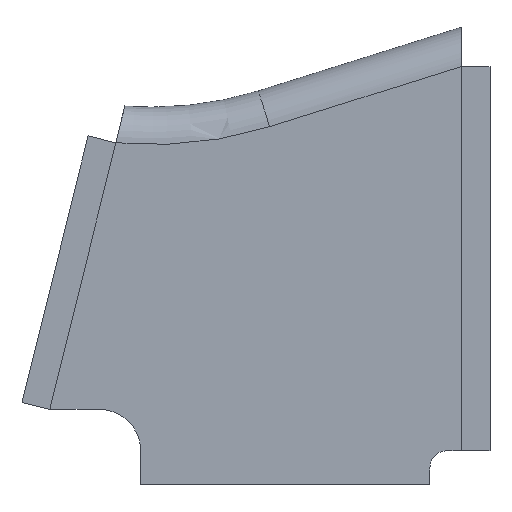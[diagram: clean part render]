
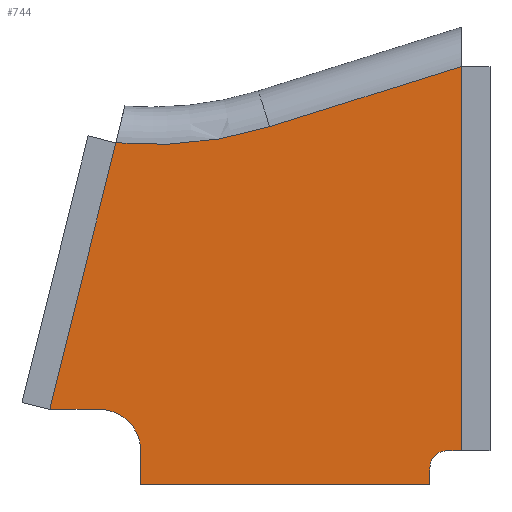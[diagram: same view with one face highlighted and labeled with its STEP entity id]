
A CAD part, front view. The second image highlights one B-rep face of the part: STEP entity #744.
In plain terms, the highlighted planar face has unit normal (0, -1, 0).
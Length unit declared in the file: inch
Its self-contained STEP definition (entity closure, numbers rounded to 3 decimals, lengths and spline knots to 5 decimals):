
#8 = CARTESIAN_POINT ( 'NONE',  ( 0.16386, 0., -3.5792 ) ) ;
#11 = CARTESIAN_POINT ( 'NONE',  ( 3.19927, 0., -3.97455 ) ) ;
#14 = LINE ( 'NONE', #32, #775 ) ;
#19 = DIRECTION ( 'NONE',  ( 0., 0., -1. ) ) ;
#20 = LINE ( 'NONE', #21, #785 ) ;
#21 = CARTESIAN_POINT ( 'NONE',  ( 0., 0., -3.97455 ) ) ;
#23 = CARTESIAN_POINT ( 'NONE',  ( -0.31259, 0., -3.18386 ) ) ;
#27 = LINE ( 'NONE', #37, #770 ) ;
#28 = DIRECTION ( 'NONE',  ( 1., 0., 0. ) ) ;
#32 = CARTESIAN_POINT ( 'NONE',  ( 0.16386, 0., 0. ) ) ;
#33 = CARTESIAN_POINT ( 'NONE',  ( -0.78905, 0., -3.18386 ) ) ;
#37 = CARTESIAN_POINT ( 'NONE',  ( 0., 0., -3.18386 ) ) ;
#40 = DIRECTION ( 'NONE',  ( 0., 1., 0. ) ) ;
#43 = DIRECTION ( 'NONE',  ( 1., 0., 0. ) ) ;
#44 = LINE ( 'NONE', #68, #783 ) ;
#51 = DIRECTION ( 'NONE',  ( 0., 0., 1. ) ) ;
#57 = CARTESIAN_POINT ( 'NONE',  ( -0.27204, 0., -3.61976 ) ) ;
#65 = CARTESIAN_POINT ( 'NONE',  ( 3.37051, 0., -3.791 ) ) ;
#66 = DIRECTION ( 'NONE',  ( 0., 0., 1. ) ) ;
#68 = CARTESIAN_POINT ( 'NONE',  ( 3.19927, 0., 0. ) ) ;
#79 = CARTESIAN_POINT ( 'NONE',  ( 0., 0., 0. ) ) ;
#83 = LINE ( 'NONE', #79, #784 ) ;
#86 = DIRECTION ( 'NONE',  ( -0.241, 0., -0.971 ) ) ;
#93 = DIRECTION ( 'NONE',  ( 0., 0., 1. ) ) ;
#100 = DIRECTION ( 'NONE',  ( 0., -1., 0. ) ) ;
#141 = LINE ( 'NONE', #151, #795 ) ;
#142 = DIRECTION ( 'NONE',  ( -0.954, 0., -0.299 ) ) ;
#148 = DIRECTION ( 'NONE',  ( 0., 1., 0. ) ) ;
#151 = CARTESIAN_POINT ( 'NONE',  ( 0.1982, 0., -0.63165 ) ) ;
#153 = CARTESIAN_POINT ( 'NONE',  ( 0.293, 0., 3.68369 ) ) ;
#159 = DIRECTION ( 'NONE',  ( 0., 0., 1. ) ) ;
#230 = CARTESIAN_POINT ( 'NONE',  ( 0., 0., -3.61976 ) ) ;
#232 = LINE ( 'NONE', #260, #855 ) ;
#244 = LINE ( 'NONE', #230, #815 ) ;
#254 = DIRECTION ( 'NONE',  ( 0., 0., -1. ) ) ;
#257 = DIRECTION ( 'NONE',  ( 1., 0., 0. ) ) ;
#260 = CARTESIAN_POINT ( 'NONE',  ( 3.52943, 0., 0. ) ) ;
#331 = PLANE ( 'NONE',  #862 ) ;
#332 = CARTESIAN_POINT ( 'NONE',  ( 0., 0., 0. ) ) ;
#337 = DIRECTION ( 'NONE',  ( 0., 0., 1. ) ) ;
#340 = DIRECTION ( 'NONE',  ( 0., 1., 0. ) ) ;
#454 = ORIENTED_EDGE ( 'NONE', *, *, #713, .T. ) ;
#459 = ORIENTED_EDGE ( 'NONE', *, *, #717, .F. ) ;
#463 = ORIENTED_EDGE ( 'NONE', *, *, #676, .F. ) ;
#469 = ORIENTED_EDGE ( 'NONE', *, *, #674, .T. ) ;
#472 = ORIENTED_EDGE ( 'NONE', *, *, #667, .T. ) ;
#474 = ORIENTED_EDGE ( 'NONE', *, *, #657, .T. ) ;
#475 = ORIENTED_EDGE ( 'NONE', *, *, #659, .T. ) ;
#477 = ORIENTED_EDGE ( 'NONE', *, *, #661, .T. ) ;
#494 = ORIENTED_EDGE ( 'NONE', *, *, #689, .T. ) ;
#496 = ORIENTED_EDGE ( 'NONE', *, *, #654, .T. ) ;
#497 = ORIENTED_EDGE ( 'NONE', *, *, #690, .T. ) ;
#554 = VERTEX_POINT ( 'NONE', #637 ) ;
#555 = VERTEX_POINT ( 'NONE', #638 ) ;
#565 = VERTEX_POINT ( 'NONE', #632 ) ;
#568 = VERTEX_POINT ( 'NONE', #646 ) ;
#573 = VERTEX_POINT ( 'NONE', #651 ) ;
#575 = VERTEX_POINT ( 'NONE', #640 ) ;
#577 = VERTEX_POINT ( 'NONE', #652 ) ;
#590 = VERTEX_POINT ( 'NONE', #33 ) ;
#594 = VERTEX_POINT ( 'NONE', #8 ) ;
#600 = VERTEX_POINT ( 'NONE', #23 ) ;
#603 = VERTEX_POINT ( 'NONE', #11 ) ;
#632 = CARTESIAN_POINT ( 'NONE',  ( 3.52943, 0., -3.61976 ) ) ;
#633 = EDGE_LOOP ( 'NONE', ( #459, #497, #494, #469, #496, #472, #474, #475, #477, #463, #454 ) ) ;
#637 = CARTESIAN_POINT ( 'NONE',  ( 3.52943, 0., 0.41361 ) ) ;
#638 = CARTESIAN_POINT ( 'NONE',  ( 0.16386, 0., -3.97455 ) ) ;
#640 = CARTESIAN_POINT ( 'NONE',  ( 3.36435, 0., -3.61976 ) ) ;
#646 = CARTESIAN_POINT ( 'NONE',  ( -0.09586, 0., -0.3868 ) ) ;
#651 = CARTESIAN_POINT ( 'NONE',  ( 1.51719, 0., -0.21778 ) ) ;
#652 = CARTESIAN_POINT ( 'NONE',  ( 3.19927, 0., -3.79715 ) ) ;
#654 = EDGE_CURVE ( 'NONE', #590, #600, #27, .T. ) ;
#657 = EDGE_CURVE ( 'NONE', #594, #555, #14, .T. ) ;
#659 = EDGE_CURVE ( 'NONE', #555, #603, #20, .T. ) ;
#661 = EDGE_CURVE ( 'NONE', #603, #577, #44, .T. ) ;
#667 = EDGE_CURVE ( 'NONE', #600, #594, #755, .T. ) ;
#674 = EDGE_CURVE ( 'NONE', #568, #590, #83, .T. ) ;
#676 = EDGE_CURVE ( 'NONE', #575, #577, #762, .T. ) ;
#689 = EDGE_CURVE ( 'NONE', #573, #568, #765, .T. ) ;
#690 = EDGE_CURVE ( 'NONE', #554, #573, #141, .T. ) ;
#713 = EDGE_CURVE ( 'NONE', #575, #565, #244, .T. ) ;
#717 = EDGE_CURVE ( 'NONE', #554, #565, #232, .T. ) ;
#744 = ADVANCED_FACE ( 'NONE', ( #876 ), #331, .F. ) ;
#755 = CIRCLE ( 'NONE', #790, 0.43778 ) ;
#762 = CIRCLE ( 'NONE', #788, 0.17135 ) ;
#765 = CIRCLE ( 'NONE', #808, 4.08903 ) ;
#770 = VECTOR ( 'NONE', #28, 39.37008 ) ;
#775 = VECTOR ( 'NONE', #19, 39.37008 ) ;
#783 = VECTOR ( 'NONE', #66, 39.37008 ) ;
#784 = VECTOR ( 'NONE', #86, 39.37008 ) ;
#785 = VECTOR ( 'NONE', #43, 39.37008 ) ;
#788 = AXIS2_PLACEMENT_3D ( 'NONE', #65, #100, #93 ) ;
#790 = AXIS2_PLACEMENT_3D ( 'NONE', #57, #40, #51 ) ;
#795 = VECTOR ( 'NONE', #142, 39.37008 ) ;
#808 = AXIS2_PLACEMENT_3D ( 'NONE', #153, #148, #159 ) ;
#815 = VECTOR ( 'NONE', #257, 39.37008 ) ;
#855 = VECTOR ( 'NONE', #254, 39.37008 ) ;
#862 = AXIS2_PLACEMENT_3D ( 'NONE', #332, #340, #337 ) ;
#876 = FACE_OUTER_BOUND ( 'NONE', #633, .T. ) ;
